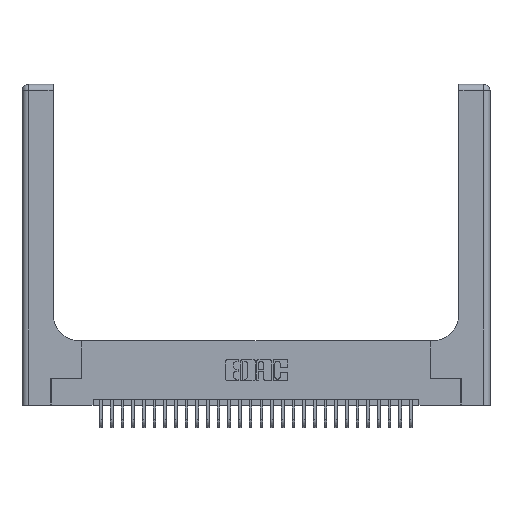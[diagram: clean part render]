
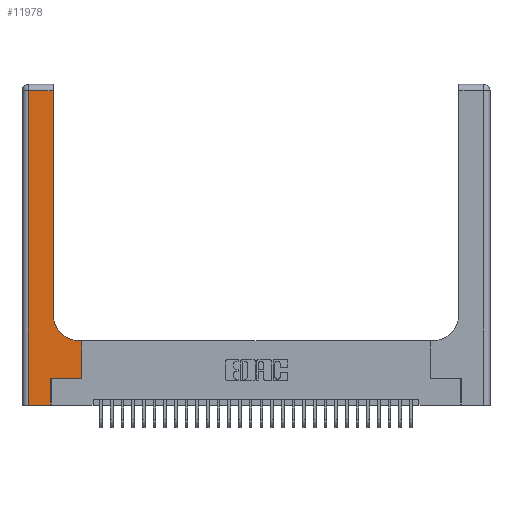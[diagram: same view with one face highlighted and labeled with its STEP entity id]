
A CAD part, top view. The second image highlights one B-rep face of the part: STEP entity #11978.
In plain terms, the highlighted planar face has unit normal (0, 0, 1).
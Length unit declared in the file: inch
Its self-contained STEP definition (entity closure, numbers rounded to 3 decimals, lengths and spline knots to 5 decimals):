
#26 = VECTOR ( 'NONE', #369, 39.37008 ) ;
#369 = DIRECTION ( 'NONE',  ( 0., 1., 0. ) ) ;
#503 = VERTEX_POINT ( 'NONE', #2164 ) ;
#1183 = ORIENTED_EDGE ( 'NONE', *, *, #16315, .T. ) ;
#1330 = FACE_OUTER_BOUND ( 'NONE', #7195, .T. ) ;
#1383 = VERTEX_POINT ( 'NONE', #27182 ) ;
#1401 = CARTESIAN_POINT ( 'NONE',  ( 0.269, 0., 0.37 ) ) ;
#2135 = VERTEX_POINT ( 'NONE', #2824 ) ;
#2164 = CARTESIAN_POINT ( 'NONE',  ( 0.2915, 2.94, 0.37 ) ) ;
#2640 = DIRECTION ( 'NONE',  ( 0., 1., 0. ) ) ;
#2824 = CARTESIAN_POINT ( 'NONE',  ( 0.06, 2.94, 0.37 ) ) ;
#3159 = VERTEX_POINT ( 'NONE', #26808 ) ;
#3927 = VECTOR ( 'NONE', #25721, 39.37008 ) ;
#4146 = CARTESIAN_POINT ( 'NONE',  ( 0., 2.94, 0.37 ) ) ;
#4151 = VECTOR ( 'NONE', #20396, 39.37008 ) ;
#4693 = VERTEX_POINT ( 'NONE', #26514 ) ;
#5156 = ORIENTED_EDGE ( 'NONE', *, *, #8524, .T. ) ;
#5307 = VECTOR ( 'NONE', #16788, 39.37008 ) ;
#5964 = VERTEX_POINT ( 'NONE', #23532 ) ;
#6142 = EDGE_CURVE ( 'NONE', #2135, #4693, #31966, .T. ) ;
#7182 = LINE ( 'NONE', #19492, #21034 ) ;
#7195 = EDGE_LOOP ( 'NONE', ( #1183, #5156, #31176, #23081, #17717, #18821, #29958, #27926, #8419 ) ) ;
#7249 = LINE ( 'NONE', #26494, #5307 ) ;
#8419 = ORIENTED_EDGE ( 'NONE', *, *, #28796, .T. ) ;
#8455 = DIRECTION ( 'NONE',  ( -1., 0., 0. ) ) ;
#8524 = EDGE_CURVE ( 'NONE', #503, #2135, #23254, .T. ) ;
#9620 = DIRECTION ( 'NONE',  ( 1., 0., 0. ) ) ;
#11081 = CARTESIAN_POINT ( 'NONE',  ( 0.2915, 0.6, 0.37 ) ) ;
#11165 = PLANE ( 'NONE',  #13406 ) ;
#11186 = VECTOR ( 'NONE', #31616, 39.37008 ) ;
#11920 = VECTOR ( 'NONE', #2640, 39.37008 ) ;
#11978 = ADVANCED_FACE ( 'NONE', ( #1330 ), #11165, .F. ) ;
#11982 = CARTESIAN_POINT ( 'NONE',  ( 0.5415, 0.85, 0.37 ) ) ;
#12086 = CARTESIAN_POINT ( 'NONE',  ( 0.06, 3., 0.37 ) ) ;
#12308 = LINE ( 'NONE', #1401, #11186 ) ;
#12800 = LINE ( 'NONE', #22702, #26 ) ;
#13044 = DIRECTION ( 'NONE',  ( 1., 0., 0. ) ) ;
#13406 = AXIS2_PLACEMENT_3D ( 'NONE', #30880, #30565, #8455 ) ;
#14563 = DIRECTION ( 'NONE',  ( 0., 0., -1. ) ) ;
#15157 = LINE ( 'NONE', #11081, #3927 ) ;
#15284 = CARTESIAN_POINT ( 'NONE',  ( 0.2915, 3., 0.37 ) ) ;
#16315 = EDGE_CURVE ( 'NONE', #5964, #503, #27352, .T. ) ;
#16352 = CARTESIAN_POINT ( 'NONE',  ( 0.5585, 0.25, 0.37 ) ) ;
#16788 = DIRECTION ( 'NONE',  ( 1., 0., 0. ) ) ;
#17717 = ORIENTED_EDGE ( 'NONE', *, *, #21416, .T. ) ;
#18821 = ORIENTED_EDGE ( 'NONE', *, *, #26904, .T. ) ;
#19373 = CARTESIAN_POINT ( 'NONE',  ( 0.5585, 0.6, 0.37 ) ) ;
#19472 = EDGE_CURVE ( 'NONE', #30529, #1383, #15157, .T. ) ;
#19492 = CARTESIAN_POINT ( 'NONE',  ( 0., 0., 0.37 ) ) ;
#19740 = EDGE_CURVE ( 'NONE', #24699, #30529, #12800, .T. ) ;
#20396 = DIRECTION ( 'NONE',  ( 0., -1., 0. ) ) ;
#21034 = VECTOR ( 'NONE', #13044, 39.37008 ) ;
#21416 = EDGE_CURVE ( 'NONE', #3159, #25234, #12308, .T. ) ;
#22702 = CARTESIAN_POINT ( 'NONE',  ( 0.5585, 0.25, 0.37 ) ) ;
#23081 = ORIENTED_EDGE ( 'NONE', *, *, #27682, .T. ) ;
#23192 = AXIS2_PLACEMENT_3D ( 'NONE', #11982, #14563, #9620 ) ;
#23254 = LINE ( 'NONE', #4146, #27941 ) ;
#23532 = CARTESIAN_POINT ( 'NONE',  ( 0.2915, 0.85, 0.37 ) ) ;
#24492 = CIRCLE ( 'NONE', #23192, 0.25 ) ;
#24699 = VERTEX_POINT ( 'NONE', #16352 ) ;
#25234 = VERTEX_POINT ( 'NONE', #25698 ) ;
#25698 = CARTESIAN_POINT ( 'NONE',  ( 0.269, 0.25, 0.37 ) ) ;
#25721 = DIRECTION ( 'NONE',  ( -1., 0., 0. ) ) ;
#26494 = CARTESIAN_POINT ( 'NONE',  ( 0.269, 0.25, 0.37 ) ) ;
#26514 = CARTESIAN_POINT ( 'NONE',  ( 0.06, 0., 0.37 ) ) ;
#26808 = CARTESIAN_POINT ( 'NONE',  ( 0.269, 0., 0.37 ) ) ;
#26904 = EDGE_CURVE ( 'NONE', #25234, #24699, #7249, .T. ) ;
#27182 = CARTESIAN_POINT ( 'NONE',  ( 0.5415, 0.6, 0.37 ) ) ;
#27352 = LINE ( 'NONE', #15284, #11920 ) ;
#27682 = EDGE_CURVE ( 'NONE', #4693, #3159, #7182, .T. ) ;
#27926 = ORIENTED_EDGE ( 'NONE', *, *, #19472, .T. ) ;
#27941 = VECTOR ( 'NONE', #28764, 39.37008 ) ;
#28764 = DIRECTION ( 'NONE',  ( -1., 0., 0. ) ) ;
#28796 = EDGE_CURVE ( 'NONE', #1383, #5964, #24492, .T. ) ;
#29958 = ORIENTED_EDGE ( 'NONE', *, *, #19740, .T. ) ;
#30529 = VERTEX_POINT ( 'NONE', #19373 ) ;
#30565 = DIRECTION ( 'NONE',  ( 0., 0., -1. ) ) ;
#30880 = CARTESIAN_POINT ( 'NONE',  ( 0., 3., 0.37 ) ) ;
#31176 = ORIENTED_EDGE ( 'NONE', *, *, #6142, .T. ) ;
#31616 = DIRECTION ( 'NONE',  ( 0., 1., 0. ) ) ;
#31966 = LINE ( 'NONE', #12086, #4151 ) ;
